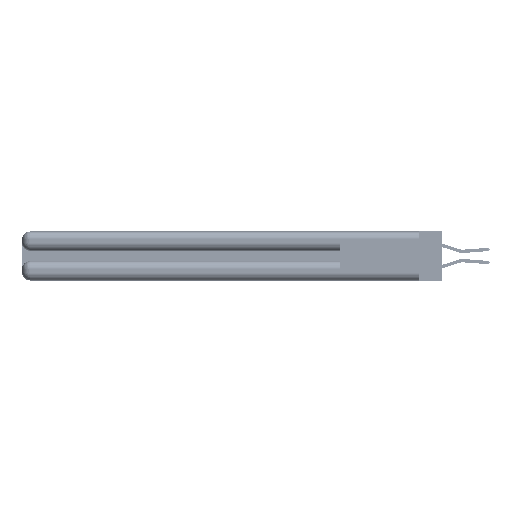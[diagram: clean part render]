
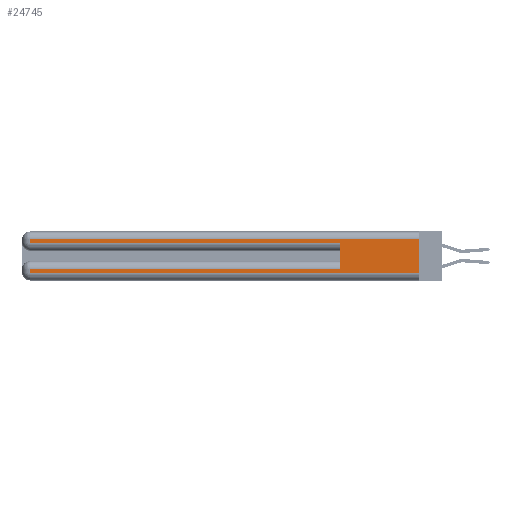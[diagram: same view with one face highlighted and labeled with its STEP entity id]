
A CAD part, left-side view. The second image highlights one B-rep face of the part: STEP entity #24745.
In plain terms, the highlighted planar face has unit normal (-1, 0, 0).
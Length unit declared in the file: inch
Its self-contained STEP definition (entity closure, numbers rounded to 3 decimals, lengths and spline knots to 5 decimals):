
#1055 = DIRECTION ( 'NONE',  ( 0., 1., 0. ) ) ;
#1767 = VERTEX_POINT ( 'NONE', #19997 ) ;
#1859 = CARTESIAN_POINT ( 'NONE',  ( 0., 2.94, 0.37 ) ) ;
#2664 = LINE ( 'NONE', #17845, #24206 ) ;
#3007 = DIRECTION ( 'NONE',  ( 0., 0., -1. ) ) ;
#3566 = EDGE_CURVE ( 'NONE', #39256, #29666, #36181, .T. ) ;
#3762 = EDGE_LOOP ( 'NONE', ( #29503, #11974, #16960, #12377, #51056, #25604, #50687, #41069 ) ) ;
#3813 = DIRECTION ( 'NONE',  ( 0., 0., -1. ) ) ;
#4068 = CARTESIAN_POINT ( 'NONE',  ( 0., 0., 0.31 ) ) ;
#4947 = DIRECTION ( 'NONE',  ( 0., -1., 0. ) ) ;
#5264 = EDGE_CURVE ( 'NONE', #26174, #40306, #52634, .T. ) ;
#5787 = CARTESIAN_POINT ( 'NONE',  ( 0., 0., 0.085 ) ) ;
#6170 = CARTESIAN_POINT ( 'NONE',  ( 0., 0., 0.37 ) ) ;
#7363 = CARTESIAN_POINT ( 'NONE',  ( 0., 2.94, 0.285 ) ) ;
#9654 = VECTOR ( 'NONE', #20048, 39.37008 ) ;
#9659 = EDGE_CURVE ( 'NONE', #40306, #53700, #20828, .T. ) ;
#10791 = CARTESIAN_POINT ( 'NONE',  ( 0., 0., 0.37 ) ) ;
#11502 = CARTESIAN_POINT ( 'NONE',  ( 0., 0.6, 0.145 ) ) ;
#11554 = CARTESIAN_POINT ( 'NONE',  ( 0., 2.94, 0.31 ) ) ;
#11974 = ORIENTED_EDGE ( 'NONE', *, *, #37925, .T. ) ;
#12200 = FACE_OUTER_BOUND ( 'NONE', #3762, .T. ) ;
#12342 = VECTOR ( 'NONE', #24028, 39.37008 ) ;
#12377 = ORIENTED_EDGE ( 'NONE', *, *, #14167, .T. ) ;
#13282 = LINE ( 'NONE', #6170, #38734 ) ;
#13427 = VECTOR ( 'NONE', #37260, 39.37008 ) ;
#13968 = VECTOR ( 'NONE', #3813, 39.37008 ) ;
#14167 = EDGE_CURVE ( 'NONE', #29666, #44833, #2664, .T. ) ;
#16374 = VECTOR ( 'NONE', #4947, 39.37008 ) ;
#16960 = ORIENTED_EDGE ( 'NONE', *, *, #3566, .T. ) ;
#17845 = CARTESIAN_POINT ( 'NONE',  ( 0., 0., 0.285 ) ) ;
#18034 = VERTEX_POINT ( 'NONE', #4068 ) ;
#19505 = PLANE ( 'NONE',  #35243 ) ;
#19997 = CARTESIAN_POINT ( 'NONE',  ( 0., 0., 0.06 ) ) ;
#20048 = DIRECTION ( 'NONE',  ( 0., 0., 1. ) ) ;
#20828 = LINE ( 'NONE', #49038, #12342 ) ;
#21919 = VECTOR ( 'NONE', #1055, 39.37008 ) ;
#22137 = CARTESIAN_POINT ( 'NONE',  ( 0., 0.6, 0.285 ) ) ;
#22222 = CARTESIAN_POINT ( 'NONE',  ( 0., 2.94, 0.085 ) ) ;
#24028 = DIRECTION ( 'NONE',  ( 0., 0., -1. ) ) ;
#24206 = VECTOR ( 'NONE', #42831, 39.37008 ) ;
#24745 = ADVANCED_FACE ( 'NONE', ( #12200 ), #19505, .F. ) ;
#25604 = ORIENTED_EDGE ( 'NONE', *, *, #5264, .T. ) ;
#26174 = VERTEX_POINT ( 'NONE', #26448 ) ;
#26448 = CARTESIAN_POINT ( 'NONE',  ( 0., 0.6, 0.085 ) ) ;
#27496 = LINE ( 'NONE', #50302, #16374 ) ;
#27737 = DIRECTION ( 'NONE',  ( 1., 0., 0. ) ) ;
#29503 = ORIENTED_EDGE ( 'NONE', *, *, #50595, .F. ) ;
#29666 = VERTEX_POINT ( 'NONE', #7363 ) ;
#30494 = LINE ( 'NONE', #11502, #9654 ) ;
#30870 = DIRECTION ( 'NONE',  ( 0., 0., -1. ) ) ;
#35243 = AXIS2_PLACEMENT_3D ( 'NONE', #10791, #27737, #3007 ) ;
#35628 = EDGE_CURVE ( 'NONE', #53700, #1767, #27496, .T. ) ;
#35646 = LINE ( 'NONE', #45839, #13427 ) ;
#36181 = LINE ( 'NONE', #1859, #13968 ) ;
#37260 = DIRECTION ( 'NONE',  ( 0., 1., 0. ) ) ;
#37925 = EDGE_CURVE ( 'NONE', #18034, #39256, #35646, .T. ) ;
#38734 = VECTOR ( 'NONE', #30870, 39.37008 ) ;
#39256 = VERTEX_POINT ( 'NONE', #11554 ) ;
#40306 = VERTEX_POINT ( 'NONE', #22222 ) ;
#41069 = ORIENTED_EDGE ( 'NONE', *, *, #35628, .T. ) ;
#42831 = DIRECTION ( 'NONE',  ( 0., -1., 0. ) ) ;
#43785 = CARTESIAN_POINT ( 'NONE',  ( 0., 2.94, 0.06 ) ) ;
#44833 = VERTEX_POINT ( 'NONE', #22137 ) ;
#45839 = CARTESIAN_POINT ( 'NONE',  ( 0., 0., 0.31 ) ) ;
#49038 = CARTESIAN_POINT ( 'NONE',  ( 0., 2.94, 0.37 ) ) ;
#50302 = CARTESIAN_POINT ( 'NONE',  ( 0., 0., 0.06 ) ) ;
#50595 = EDGE_CURVE ( 'NONE', #18034, #1767, #13282, .T. ) ;
#50687 = ORIENTED_EDGE ( 'NONE', *, *, #9659, .T. ) ;
#51056 = ORIENTED_EDGE ( 'NONE', *, *, #53951, .F. ) ;
#52634 = LINE ( 'NONE', #5787, #21919 ) ;
#53700 = VERTEX_POINT ( 'NONE', #43785 ) ;
#53951 = EDGE_CURVE ( 'NONE', #26174, #44833, #30494, .T. ) ;
